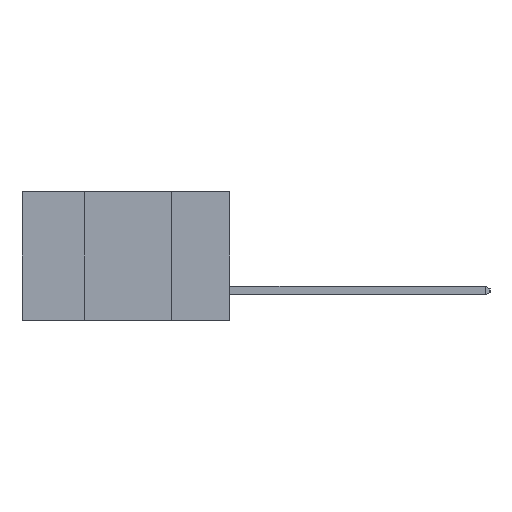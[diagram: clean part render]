
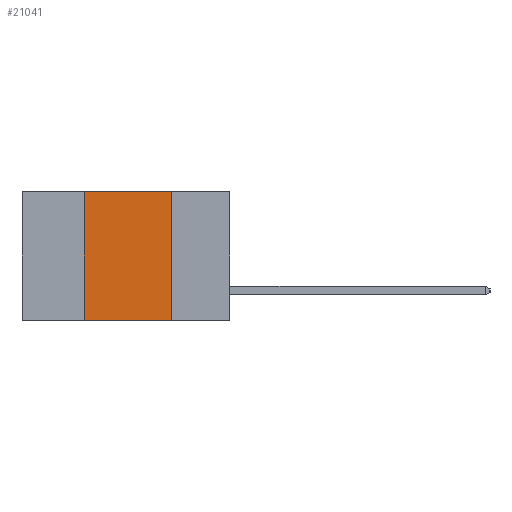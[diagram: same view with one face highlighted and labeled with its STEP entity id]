
A CAD part, left-side view. The second image highlights one B-rep face of the part: STEP entity #21041.
In plain terms, the highlighted planar face has unit normal (-1, 0, 0).
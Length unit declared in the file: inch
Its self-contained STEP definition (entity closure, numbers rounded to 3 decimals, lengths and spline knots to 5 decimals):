
#28 = AXIS2_PLACEMENT_3D ( 'NONE', #21137, #3902, #17393 ) ;
#1395 = ORIENTED_EDGE ( 'NONE', *, *, #17292, .F. ) ;
#1528 = FACE_OUTER_BOUND ( 'NONE', #10912, .T. ) ;
#2317 = ORIENTED_EDGE ( 'NONE', *, *, #15073, .F. ) ;
#3893 = LINE ( 'NONE', #16675, #13584 ) ;
#3902 = DIRECTION ( 'NONE',  ( 1., 0., 0. ) ) ;
#4193 = VECTOR ( 'NONE', #17255, 39.37008 ) ;
#6193 = VERTEX_POINT ( 'NONE', #16321 ) ;
#9499 = CARTESIAN_POINT ( 'NONE',  ( 0., 0.17, -0.37 ) ) ;
#9629 = PLANE ( 'NONE',  #28 ) ;
#10477 = VECTOR ( 'NONE', #13500, 39.37008 ) ;
#10912 = EDGE_LOOP ( 'NONE', ( #19157, #2317, #1395, #16147 ) ) ;
#11085 = VECTOR ( 'NONE', #24527, 39.37008 ) ;
#11159 = CARTESIAN_POINT ( 'NONE',  ( 0., 0.6, 0. ) ) ;
#11361 = VERTEX_POINT ( 'NONE', #21417 ) ;
#11555 = VERTEX_POINT ( 'NONE', #18242 ) ;
#13500 = DIRECTION ( 'NONE',  ( 0., 0., 1. ) ) ;
#13584 = VECTOR ( 'NONE', #20513, 39.37008 ) ;
#13690 = EDGE_CURVE ( 'NONE', #11361, #6193, #3893, .T. ) ;
#13877 = EDGE_CURVE ( 'NONE', #21904, #6193, #14475, .T. ) ;
#14475 = LINE ( 'NONE', #9499, #4193 ) ;
#15011 = LINE ( 'NONE', #24895, #10477 ) ;
#15073 = EDGE_CURVE ( 'NONE', #11555, #21904, #21271, .T. ) ;
#16147 = ORIENTED_EDGE ( 'NONE', *, *, #13690, .T. ) ;
#16321 = CARTESIAN_POINT ( 'NONE',  ( 0., 0.17, -0.37 ) ) ;
#16675 = CARTESIAN_POINT ( 'NONE',  ( 0., 0.6, -0.37 ) ) ;
#17255 = DIRECTION ( 'NONE',  ( 0., 0., -1. ) ) ;
#17292 = EDGE_CURVE ( 'NONE', #11361, #11555, #15011, .T. ) ;
#17393 = DIRECTION ( 'NONE',  ( 0., 0., -1. ) ) ;
#18242 = CARTESIAN_POINT ( 'NONE',  ( 0., 0.42, 0. ) ) ;
#19157 = ORIENTED_EDGE ( 'NONE', *, *, #13877, .F. ) ;
#20513 = DIRECTION ( 'NONE',  ( 0., -1., 0. ) ) ;
#21041 = ADVANCED_FACE ( 'NONE', ( #1528 ), #9629, .F. ) ;
#21137 = CARTESIAN_POINT ( 'NONE',  ( 0., 0.6, 0. ) ) ;
#21271 = LINE ( 'NONE', #11159, #11085 ) ;
#21417 = CARTESIAN_POINT ( 'NONE',  ( 0., 0.42, -0.37 ) ) ;
#21904 = VERTEX_POINT ( 'NONE', #23591 ) ;
#23591 = CARTESIAN_POINT ( 'NONE',  ( 0., 0.17, 0. ) ) ;
#24527 = DIRECTION ( 'NONE',  ( 0., -1., 0. ) ) ;
#24895 = CARTESIAN_POINT ( 'NONE',  ( 0., 0.42, -0.37 ) ) ;
